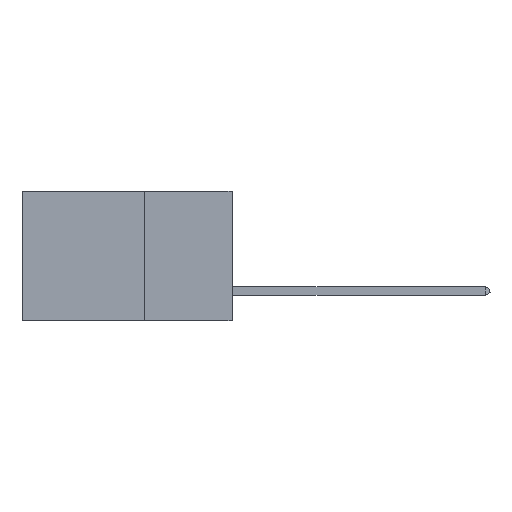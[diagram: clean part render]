
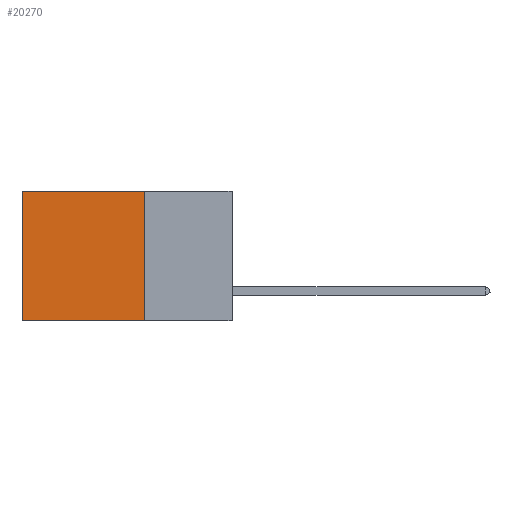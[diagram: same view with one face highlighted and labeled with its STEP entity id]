
A CAD part, left-side view. The second image highlights one B-rep face of the part: STEP entity #20270.
In plain terms, the highlighted planar face has unit normal (-1, 0, 0).
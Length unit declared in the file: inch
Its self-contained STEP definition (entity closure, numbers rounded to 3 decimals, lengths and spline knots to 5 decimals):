
#609 = VECTOR ( 'NONE', #1151, 39.37008 ) ;
#690 = PLANE ( 'NONE',  #13340 ) ;
#883 = CARTESIAN_POINT ( 'NONE',  ( 0.2875, 0.25, 0. ) ) ;
#962 = DIRECTION ( 'NONE',  ( 0., 0., -1. ) ) ;
#1151 = DIRECTION ( 'NONE',  ( 0., 0., -1. ) ) ;
#1256 = VECTOR ( 'NONE', #20800, 39.37008 ) ;
#3395 = EDGE_CURVE ( 'NONE', #12905, #16177, #21452, .T. ) ;
#3631 = CARTESIAN_POINT ( 'NONE',  ( 0.2875, 0.6, -0.37 ) ) ;
#3758 = ORIENTED_EDGE ( 'NONE', *, *, #17956, .T. ) ;
#4060 = EDGE_LOOP ( 'NONE', ( #21356, #11567, #9877, #3758 ) ) ;
#5155 = LINE ( 'NONE', #17243, #1256 ) ;
#5720 = VERTEX_POINT ( 'NONE', #14888 ) ;
#8201 = LINE ( 'NONE', #883, #16182 ) ;
#8720 = VECTOR ( 'NONE', #17115, 39.37008 ) ;
#9877 = ORIENTED_EDGE ( 'NONE', *, *, #3395, .F. ) ;
#11567 = ORIENTED_EDGE ( 'NONE', *, *, #14132, .F. ) ;
#11587 = DIRECTION ( 'NONE',  ( 0., 1., 0. ) ) ;
#12905 = VERTEX_POINT ( 'NONE', #19491 ) ;
#13340 = AXIS2_PLACEMENT_3D ( 'NONE', #16301, #22499, #962 ) ;
#14132 = EDGE_CURVE ( 'NONE', #16177, #19358, #17002, .T. ) ;
#14193 = FACE_OUTER_BOUND ( 'NONE', #4060, .T. ) ;
#14888 = CARTESIAN_POINT ( 'NONE',  ( 0.2875, 0.6, 0. ) ) ;
#15996 = CARTESIAN_POINT ( 'NONE',  ( 0.2875, 0.25, -0.37 ) ) ;
#16177 = VERTEX_POINT ( 'NONE', #15996 ) ;
#16182 = VECTOR ( 'NONE', #11587, 39.37008 ) ;
#16301 = CARTESIAN_POINT ( 'NONE',  ( 0.2875, 0.25, 0. ) ) ;
#17002 = LINE ( 'NONE', #20475, #8720 ) ;
#17115 = DIRECTION ( 'NONE',  ( 0., 1., 0. ) ) ;
#17243 = CARTESIAN_POINT ( 'NONE',  ( 0.2875, 0.6, 0. ) ) ;
#17956 = EDGE_CURVE ( 'NONE', #12905, #5720, #8201, .T. ) ;
#18312 = EDGE_CURVE ( 'NONE', #5720, #19358, #5155, .T. ) ;
#19358 = VERTEX_POINT ( 'NONE', #3631 ) ;
#19491 = CARTESIAN_POINT ( 'NONE',  ( 0.2875, 0.25, 0. ) ) ;
#20270 = ADVANCED_FACE ( 'NONE', ( #14193 ), #690, .F. ) ;
#20475 = CARTESIAN_POINT ( 'NONE',  ( 0.2875, 0.25, -0.37 ) ) ;
#20800 = DIRECTION ( 'NONE',  ( 0., 0., -1. ) ) ;
#21356 = ORIENTED_EDGE ( 'NONE', *, *, #18312, .T. ) ;
#21452 = LINE ( 'NONE', #22170, #609 ) ;
#22170 = CARTESIAN_POINT ( 'NONE',  ( 0.2875, 0.25, 0. ) ) ;
#22499 = DIRECTION ( 'NONE',  ( 1., 0., 0. ) ) ;
